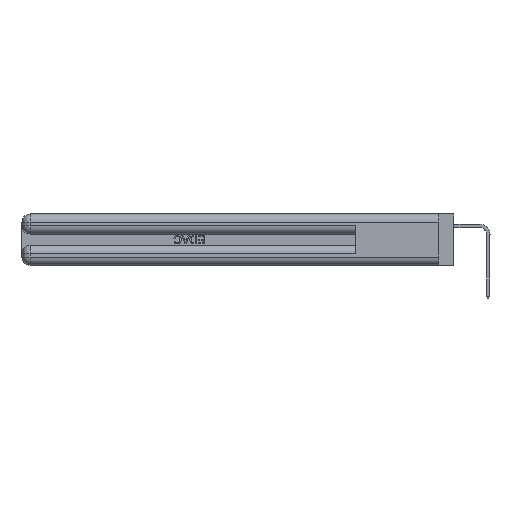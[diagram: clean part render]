
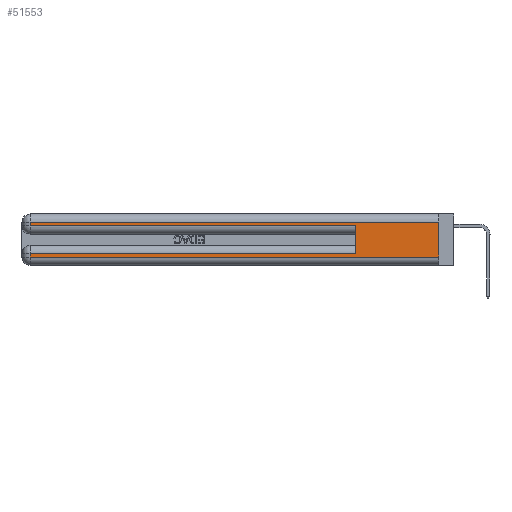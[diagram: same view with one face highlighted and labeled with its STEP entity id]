
A CAD part, left-side view. The second image highlights one B-rep face of the part: STEP entity #51553.
In plain terms, the highlighted planar face has unit normal (-1, 0, 0).
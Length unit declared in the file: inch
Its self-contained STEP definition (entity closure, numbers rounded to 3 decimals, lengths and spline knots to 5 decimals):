
#1184 = LINE ( 'NONE', #29604, #53654 ) ;
#2551 = VERTEX_POINT ( 'NONE', #26374 ) ;
#3052 = CARTESIAN_POINT ( 'NONE',  ( 0., 0., 0.285 ) ) ;
#4354 = CARTESIAN_POINT ( 'NONE',  ( 0., 0., 0.37 ) ) ;
#4434 = ORIENTED_EDGE ( 'NONE', *, *, #51928, .T. ) ;
#5270 = EDGE_CURVE ( 'NONE', #29653, #2551, #8230, .T. ) ;
#5425 = CARTESIAN_POINT ( 'NONE',  ( 0., 0., 0.31 ) ) ;
#5625 = LINE ( 'NONE', #34056, #48365 ) ;
#7018 = DIRECTION ( 'NONE',  ( 0., 0., -1. ) ) ;
#7856 = CARTESIAN_POINT ( 'NONE',  ( 0., 0., 0.06 ) ) ;
#8230 = LINE ( 'NONE', #3052, #28915 ) ;
#8975 = DIRECTION ( 'NONE',  ( 0., 0., 1. ) ) ;
#9896 = LINE ( 'NONE', #49719, #11201 ) ;
#10601 = EDGE_LOOP ( 'NONE', ( #47989, #53108, #4434, #23695, #11641, #35312, #12716, #31684 ) ) ;
#11201 = VECTOR ( 'NONE', #24952, 39.37008 ) ;
#11641 = ORIENTED_EDGE ( 'NONE', *, *, #17741, .F. ) ;
#12345 = VECTOR ( 'NONE', #26310, 39.37008 ) ;
#12716 = ORIENTED_EDGE ( 'NONE', *, *, #46464, .T. ) ;
#13831 = CARTESIAN_POINT ( 'NONE',  ( 0., 0., 0.37 ) ) ;
#16065 = CARTESIAN_POINT ( 'NONE',  ( 0., 0., 0.085 ) ) ;
#16802 = DIRECTION ( 'NONE',  ( 0., 0., -1. ) ) ;
#17741 = EDGE_CURVE ( 'NONE', #50752, #2551, #1184, .T. ) ;
#17971 = DIRECTION ( 'NONE',  ( 0., 0., -1. ) ) ;
#18343 = CARTESIAN_POINT ( 'NONE',  ( 0., 0.6, 0.085 ) ) ;
#18505 = CARTESIAN_POINT ( 'NONE',  ( 0., 2.94, 0.085 ) ) ;
#20863 = VERTEX_POINT ( 'NONE', #18505 ) ;
#20886 = CARTESIAN_POINT ( 'NONE',  ( 0., 2.94, 0.31 ) ) ;
#23178 = CARTESIAN_POINT ( 'NONE',  ( 0., 2.94, 0.285 ) ) ;
#23695 = ORIENTED_EDGE ( 'NONE', *, *, #5270, .T. ) ;
#24952 = DIRECTION ( 'NONE',  ( 0., 0., -1. ) ) ;
#25869 = LINE ( 'NONE', #16065, #35575 ) ;
#26310 = DIRECTION ( 'NONE',  ( 0., -1., 0. ) ) ;
#26374 = CARTESIAN_POINT ( 'NONE',  ( 0., 0.6, 0.285 ) ) ;
#27490 = VECTOR ( 'NONE', #17971, 39.37008 ) ;
#28557 = AXIS2_PLACEMENT_3D ( 'NONE', #4354, #41592, #16802 ) ;
#28915 = VECTOR ( 'NONE', #40133, 39.37008 ) ;
#28930 = PLANE ( 'NONE',  #28557 ) ;
#29604 = CARTESIAN_POINT ( 'NONE',  ( 0., 0.6, 0.145 ) ) ;
#29653 = VERTEX_POINT ( 'NONE', #23178 ) ;
#30120 = VERTEX_POINT ( 'NONE', #5425 ) ;
#30327 = EDGE_CURVE ( 'NONE', #50752, #20863, #25869, .T. ) ;
#31028 = VERTEX_POINT ( 'NONE', #20886 ) ;
#31684 = ORIENTED_EDGE ( 'NONE', *, *, #50701, .T. ) ;
#31804 = CARTESIAN_POINT ( 'NONE',  ( 0., 2.94, 0.37 ) ) ;
#34056 = CARTESIAN_POINT ( 'NONE',  ( 0., 0., 0.31 ) ) ;
#34059 = CARTESIAN_POINT ( 'NONE',  ( 0., 2.94, 0.06 ) ) ;
#35312 = ORIENTED_EDGE ( 'NONE', *, *, #30327, .T. ) ;
#35550 = FACE_OUTER_BOUND ( 'NONE', #10601, .T. ) ;
#35575 = VECTOR ( 'NONE', #45043, 39.37008 ) ;
#38678 = VERTEX_POINT ( 'NONE', #34059 ) ;
#40133 = DIRECTION ( 'NONE',  ( 0., -1., 0. ) ) ;
#41409 = VECTOR ( 'NONE', #7018, 39.37008 ) ;
#41592 = DIRECTION ( 'NONE',  ( 1., 0., 0. ) ) ;
#41854 = VERTEX_POINT ( 'NONE', #7856 ) ;
#42584 = CARTESIAN_POINT ( 'NONE',  ( 0., 0., 0.06 ) ) ;
#44171 = EDGE_CURVE ( 'NONE', #30120, #31028, #5625, .T. ) ;
#45043 = DIRECTION ( 'NONE',  ( 0., 1., 0. ) ) ;
#45380 = LINE ( 'NONE', #42584, #12345 ) ;
#45460 = EDGE_CURVE ( 'NONE', #30120, #41854, #49477, .T. ) ;
#46464 = EDGE_CURVE ( 'NONE', #20863, #38678, #9896, .T. ) ;
#47989 = ORIENTED_EDGE ( 'NONE', *, *, #45460, .F. ) ;
#48365 = VECTOR ( 'NONE', #50850, 39.37008 ) ;
#49477 = LINE ( 'NONE', #13831, #27490 ) ;
#49719 = CARTESIAN_POINT ( 'NONE',  ( 0., 2.94, 0.37 ) ) ;
#50701 = EDGE_CURVE ( 'NONE', #38678, #41854, #45380, .T. ) ;
#50752 = VERTEX_POINT ( 'NONE', #18343 ) ;
#50850 = DIRECTION ( 'NONE',  ( 0., 1., 0. ) ) ;
#51109 = LINE ( 'NONE', #31804, #41409 ) ;
#51553 = ADVANCED_FACE ( 'NONE', ( #35550 ), #28930, .F. ) ;
#51928 = EDGE_CURVE ( 'NONE', #31028, #29653, #51109, .T. ) ;
#53108 = ORIENTED_EDGE ( 'NONE', *, *, #44171, .T. ) ;
#53654 = VECTOR ( 'NONE', #8975, 39.37008 ) ;
